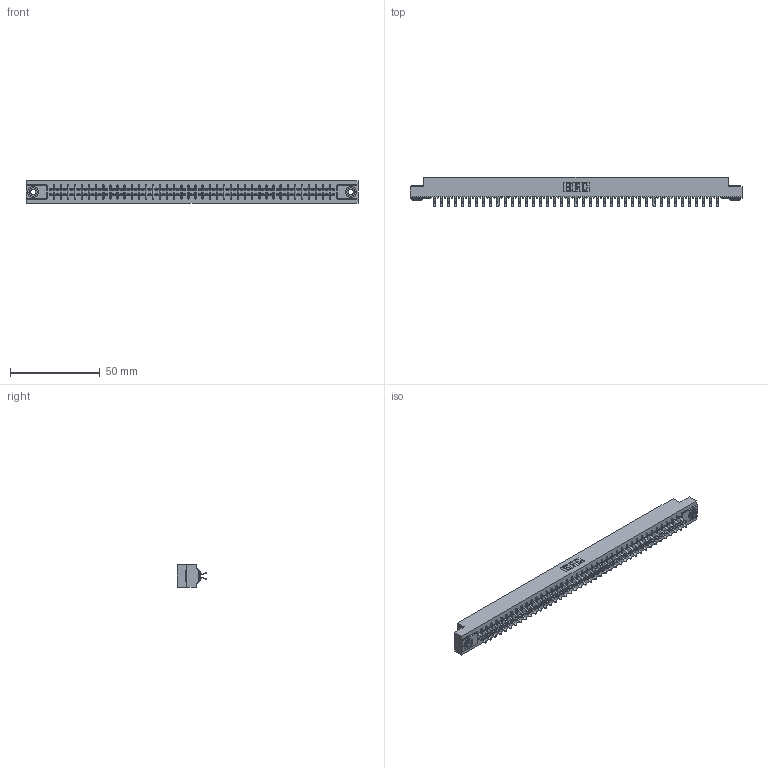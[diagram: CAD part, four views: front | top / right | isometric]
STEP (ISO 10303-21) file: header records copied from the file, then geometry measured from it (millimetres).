
FILE_DESCRIPTION (( 'STEP AP203' ), '1' );
FILE_NAME ('315-082-556-203.STEP', '2019-09-10T23:41:09', ( '' ), ( '' ), 'SwSTEP 2.0', 'SolidWorks 2016', '' );
FILE_SCHEMA (( 'CONFIG_CONTROL_DESIGN' ));
Length unit declared in the file: inch
Products named in the file (4): 345-250-002_345-250-002-102; 305-290-001_556; 305 Part_.156 Dia; 315-082-556-203
Assembly tree (85 placements, depth 2):
  315-082-556-203
    305 Part_.156 Dia
    305-290-001_556  x82
    345-250-002_345-250-002-102  x2
Bounding box: 185.47 x 16.64 x 12.7 mm (x, y, z)
Volume: 19333.4 mm3; surface area: 24847.3 mm2
Topology: 85 solids, 85 shells, 4760 faces, 13671 edges, 8890 vertices
Faces by surface type: plane 2634, cylinder 1954, sphere 164, cone 8
Entity records: 45801 total; most frequent: CARTESIAN_POINT 7562, ORIENTED_EDGE 7498, DIRECTION 7335, EDGE_CURVE 3749, LINE 3017, VECTOR 3017, VERTEX_POINT 2386, AXIS2_PLACEMENT_3D 2159
